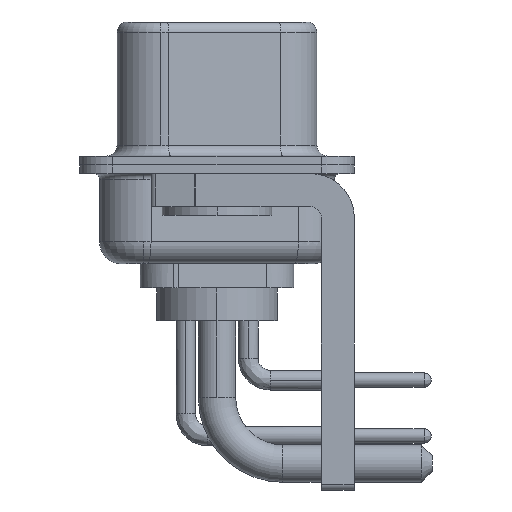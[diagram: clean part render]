
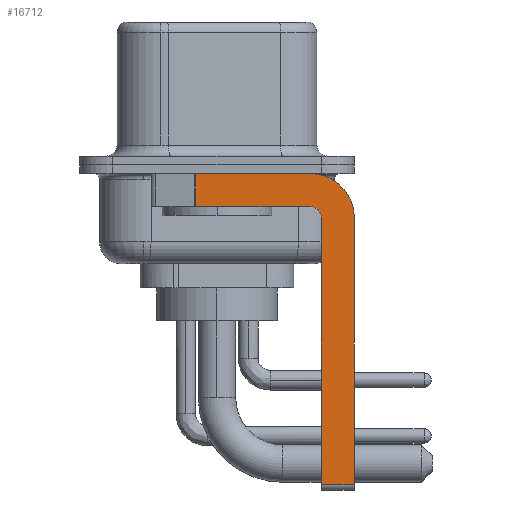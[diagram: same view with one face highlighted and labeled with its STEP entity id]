
A CAD part, left-side view. The second image highlights one B-rep face of the part: STEP entity #16712.
In plain terms, the highlighted planar face has unit normal (-1, 0, 0).
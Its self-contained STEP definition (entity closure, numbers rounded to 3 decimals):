
#326 = CARTESIAN_POINT ( 'NONE',  ( -2.9, -4.75, -2.4 ) ) ;
#912 = ORIENTED_EDGE ( 'NONE', *, *, #14913, .F. ) ;
#956 = CARTESIAN_POINT ( 'NONE',  ( -2.9, -4.25, -0.4 ) ) ;
#1026 = AXIS2_PLACEMENT_3D ( 'NONE', #10256, #1911, #6407 ) ;
#1123 = DIRECTION ( 'NONE',  ( 0., 0., -1. ) ) ;
#1910 = CARTESIAN_POINT ( 'NONE',  ( -2.9, -4.75, -14.55 ) ) ;
#1911 = DIRECTION ( 'NONE',  ( -1., 0., 0. ) ) ;
#1921 = FACE_OUTER_BOUND ( 'NONE', #18312, .T. ) ;
#2373 = VECTOR ( 'NONE', #16877, 1000. ) ;
#2885 = CARTESIAN_POINT ( 'NONE',  ( -2.9, 0.978, -1.9 ) ) ;
#3128 = CIRCLE ( 'NONE', #1026, 0.5 ) ;
#3204 = VERTEX_POINT ( 'NONE', #956 ) ;
#3466 = VECTOR ( 'NONE', #3695, 1000. ) ;
#3695 = DIRECTION ( 'NONE',  ( 0., 1., 0. ) ) ;
#3779 = DIRECTION ( 'NONE',  ( 0., 0., -1. ) ) ;
#3797 = LINE ( 'NONE', #5221, #3466 ) ;
#4019 = CARTESIAN_POINT ( 'NONE',  ( -2.9, -6.25, -2.4 ) ) ;
#4157 = ORIENTED_EDGE ( 'NONE', *, *, #17994, .F. ) ;
#4242 = EDGE_CURVE ( 'NONE', #3204, #9571, #13470, .T. ) ;
#4314 = CARTESIAN_POINT ( 'NONE',  ( -2.9, -4.25, -14.55 ) ) ;
#4342 = LINE ( 'NONE', #4019, #5543 ) ;
#4792 = CARTESIAN_POINT ( 'NONE',  ( -2.9, -6.25, -2.4 ) ) ;
#5221 = CARTESIAN_POINT ( 'NONE',  ( -2.9, -4.25, -1.9 ) ) ;
#5543 = VECTOR ( 'NONE', #20696, 1000. ) ;
#5722 = DIRECTION ( 'NONE',  ( 0., 0., -1. ) ) ;
#5730 = VECTOR ( 'NONE', #1123, 1000. ) ;
#5836 = LINE ( 'NONE', #4314, #16962 ) ;
#6407 = DIRECTION ( 'NONE',  ( 0., 0., 1. ) ) ;
#6465 = VERTEX_POINT ( 'NONE', #1910 ) ;
#7070 = LINE ( 'NONE', #7396, #15733 ) ;
#7396 = CARTESIAN_POINT ( 'NONE',  ( -2.9, -4.75, -14.8 ) ) ;
#7917 = LINE ( 'NONE', #2885, #5730 ) ;
#8073 = EDGE_CURVE ( 'NONE', #14187, #15053, #7917, .T. ) ;
#8160 = VERTEX_POINT ( 'NONE', #8463 ) ;
#8424 = EDGE_CURVE ( 'NONE', #6465, #8160, #5836, .T. ) ;
#8463 = CARTESIAN_POINT ( 'NONE',  ( -2.9, -6.25, -14.55 ) ) ;
#8987 = CARTESIAN_POINT ( 'NONE',  ( -2.9, -4.25, -1.9 ) ) ;
#9531 = ORIENTED_EDGE ( 'NONE', *, *, #8073, .T. ) ;
#9571 = VERTEX_POINT ( 'NONE', #4792 ) ;
#10256 = CARTESIAN_POINT ( 'NONE',  ( -2.9, -4.25, -2.4 ) ) ;
#10667 = AXIS2_PLACEMENT_3D ( 'NONE', #10890, #16034, #5722 ) ;
#10818 = ORIENTED_EDGE ( 'NONE', *, *, #18453, .F. ) ;
#10890 = CARTESIAN_POINT ( 'NONE',  ( -2.9, -4.25, -2.4 ) ) ;
#11737 = LINE ( 'NONE', #19952, #2373 ) ;
#13470 = CIRCLE ( 'NONE', #10667, 2. ) ;
#13483 = EDGE_CURVE ( 'NONE', #14187, #3204, #11737, .T. ) ;
#13651 = CARTESIAN_POINT ( 'NONE',  ( -2.9, -4.25, -2.4 ) ) ;
#14187 = VERTEX_POINT ( 'NONE', #16342 ) ;
#14725 = AXIS2_PLACEMENT_3D ( 'NONE', #13651, #18917, #3779 ) ;
#14741 = EDGE_CURVE ( 'NONE', #19384, #15053, #3797, .T. ) ;
#14913 = EDGE_CURVE ( 'NONE', #9571, #8160, #4342, .T. ) ;
#14973 = ORIENTED_EDGE ( 'NONE', *, *, #8424, .T. ) ;
#15053 = VERTEX_POINT ( 'NONE', #19579 ) ;
#15545 = DIRECTION ( 'NONE',  ( 0., 0., 1. ) ) ;
#15733 = VECTOR ( 'NONE', #15545, 1000. ) ;
#16034 = DIRECTION ( 'NONE',  ( 1., 0., 0. ) ) ;
#16342 = CARTESIAN_POINT ( 'NONE',  ( -2.9, 0.978, -0.4 ) ) ;
#16712 = ADVANCED_FACE ( 'NONE', ( #1921 ), #17269, .F. ) ;
#16877 = DIRECTION ( 'NONE',  ( 0., -1., 0. ) ) ;
#16962 = VECTOR ( 'NONE', #20555, 1000. ) ;
#17269 = PLANE ( 'NONE',  #14725 ) ;
#17444 = VERTEX_POINT ( 'NONE', #326 ) ;
#17994 = EDGE_CURVE ( 'NONE', #6465, #17444, #7070, .T. ) ;
#18312 = EDGE_LOOP ( 'NONE', ( #18577, #9531, #19455, #10818, #4157, #14973, #912, #21016 ) ) ;
#18453 = EDGE_CURVE ( 'NONE', #17444, #19384, #3128, .T. ) ;
#18577 = ORIENTED_EDGE ( 'NONE', *, *, #13483, .F. ) ;
#18917 = DIRECTION ( 'NONE',  ( 1., 0., 0. ) ) ;
#19384 = VERTEX_POINT ( 'NONE', #8987 ) ;
#19455 = ORIENTED_EDGE ( 'NONE', *, *, #14741, .F. ) ;
#19579 = CARTESIAN_POINT ( 'NONE',  ( -2.9, 0.978, -1.9 ) ) ;
#19952 = CARTESIAN_POINT ( 'NONE',  ( -2.9, 3., -0.4 ) ) ;
#20555 = DIRECTION ( 'NONE',  ( 0., -1., 0. ) ) ;
#20696 = DIRECTION ( 'NONE',  ( 0., 0., -1. ) ) ;
#21016 = ORIENTED_EDGE ( 'NONE', *, *, #4242, .F. ) ;
